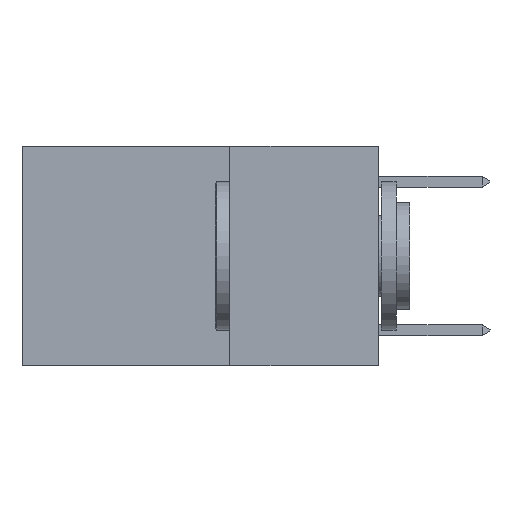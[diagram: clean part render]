
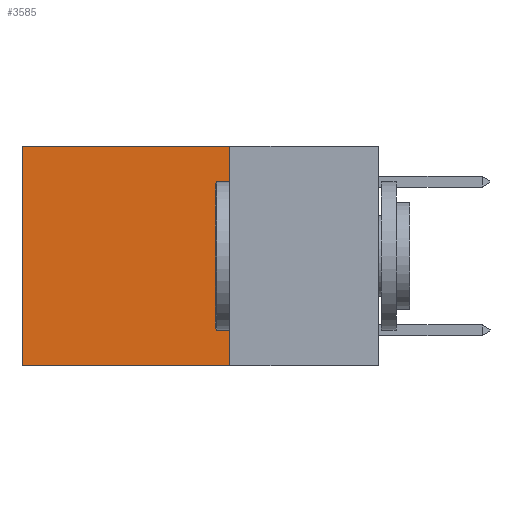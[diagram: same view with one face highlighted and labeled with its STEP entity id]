
A CAD part, left-side view. The second image highlights one B-rep face of the part: STEP entity #3585.
In plain terms, the highlighted planar face has unit normal (-1, 0, 0).
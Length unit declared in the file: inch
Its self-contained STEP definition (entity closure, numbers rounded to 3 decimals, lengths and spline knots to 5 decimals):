
#58 = CARTESIAN_POINT ( 'NONE',  ( 0.2625, 0.25, 0. ) ) ;
#91 = VERTEX_POINT ( 'NONE', #58 ) ;
#133 = CARTESIAN_POINT ( 'NONE',  ( 0.2625, 0.6, -0.37 ) ) ;
#354 = LINE ( 'NONE', #4023, #1733 ) ;
#771 = LINE ( 'NONE', #5092, #12572 ) ;
#837 = ORIENTED_EDGE ( 'NONE', *, *, #4273, .F. ) ;
#1080 = EDGE_CURVE ( 'NONE', #91, #6012, #354, .T. ) ;
#1350 = DIRECTION ( 'NONE',  ( 0., 0., -1. ) ) ;
#1374 = VECTOR ( 'NONE', #2504, 39.37008 ) ;
#1523 = VERTEX_POINT ( 'NONE', #1905 ) ;
#1733 = VECTOR ( 'NONE', #3115, 39.37008 ) ;
#1905 = CARTESIAN_POINT ( 'NONE',  ( 0.2625, 0.25, -0.37 ) ) ;
#1925 = VECTOR ( 'NONE', #1350, 39.37008 ) ;
#2105 = EDGE_CURVE ( 'NONE', #6012, #7054, #10452, .T. ) ;
#2234 = LINE ( 'NONE', #11904, #1925 ) ;
#2504 = DIRECTION ( 'NONE',  ( 0., 0., -1. ) ) ;
#3115 = DIRECTION ( 'NONE',  ( 0., 1., 0. ) ) ;
#3585 = ADVANCED_FACE ( 'NONE', ( #10480 ), #10778, .F. ) ;
#3979 = DIRECTION ( 'NONE',  ( 0., 0., -1. ) ) ;
#4023 = CARTESIAN_POINT ( 'NONE',  ( 0.2625, 0.25, 0. ) ) ;
#4273 = EDGE_CURVE ( 'NONE', #1523, #7054, #771, .T. ) ;
#5092 = CARTESIAN_POINT ( 'NONE',  ( 0.2625, 0.25, -0.37 ) ) ;
#5857 = DIRECTION ( 'NONE',  ( 1., 0., 0. ) ) ;
#5927 = EDGE_LOOP ( 'NONE', ( #6945, #837, #6662, #8142 ) ) ;
#6012 = VERTEX_POINT ( 'NONE', #8968 ) ;
#6662 = ORIENTED_EDGE ( 'NONE', *, *, #10378, .F. ) ;
#6775 = CARTESIAN_POINT ( 'NONE',  ( 0.2625, 0.25, 0. ) ) ;
#6945 = ORIENTED_EDGE ( 'NONE', *, *, #2105, .T. ) ;
#7054 = VERTEX_POINT ( 'NONE', #133 ) ;
#7523 = AXIS2_PLACEMENT_3D ( 'NONE', #6775, #5857, #3979 ) ;
#8142 = ORIENTED_EDGE ( 'NONE', *, *, #1080, .T. ) ;
#8968 = CARTESIAN_POINT ( 'NONE',  ( 0.2625, 0.6, 0. ) ) ;
#10077 = DIRECTION ( 'NONE',  ( 0., 1., 0. ) ) ;
#10378 = EDGE_CURVE ( 'NONE', #91, #1523, #2234, .T. ) ;
#10452 = LINE ( 'NONE', #11432, #1374 ) ;
#10480 = FACE_OUTER_BOUND ( 'NONE', #5927, .T. ) ;
#10778 = PLANE ( 'NONE',  #7523 ) ;
#11432 = CARTESIAN_POINT ( 'NONE',  ( 0.2625, 0.6, 0. ) ) ;
#11904 = CARTESIAN_POINT ( 'NONE',  ( 0.2625, 0.25, 0. ) ) ;
#12572 = VECTOR ( 'NONE', #10077, 39.37008 ) ;
